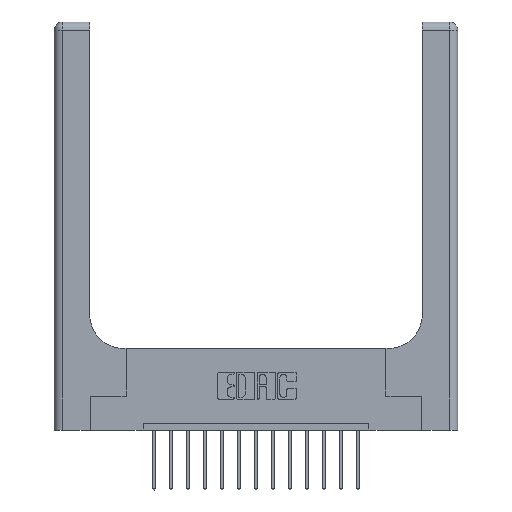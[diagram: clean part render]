
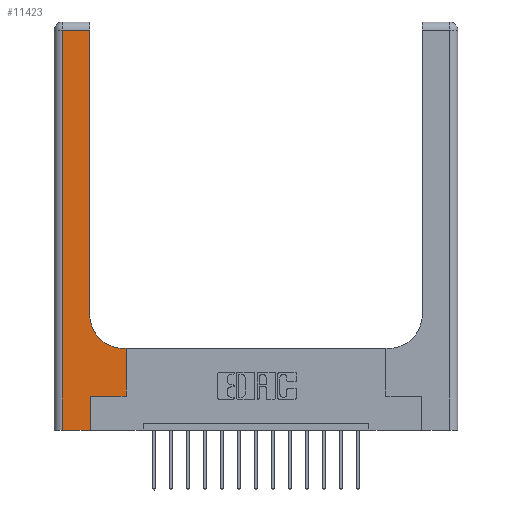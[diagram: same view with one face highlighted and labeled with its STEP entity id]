
A CAD part, top view. The second image highlights one B-rep face of the part: STEP entity #11423.
In plain terms, the highlighted planar face has unit normal (0, 0, 1).
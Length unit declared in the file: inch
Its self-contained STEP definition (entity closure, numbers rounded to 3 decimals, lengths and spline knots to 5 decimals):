
#412 = VERTEX_POINT ( 'NONE', #4691 ) ;
#681 = DIRECTION ( 'NONE',  ( 1., 0., 0. ) ) ;
#882 = LINE ( 'NONE', #3858, #10049 ) ;
#1026 = CARTESIAN_POINT ( 'NONE',  ( 0.528, 0.25, 0.37 ) ) ;
#1270 = DIRECTION ( 'NONE',  ( -1., 0., 0. ) ) ;
#1473 = ORIENTED_EDGE ( 'NONE', *, *, #4287, .T. ) ;
#1665 = DIRECTION ( 'NONE',  ( 0., 1., 0. ) ) ;
#1881 = CARTESIAN_POINT ( 'NONE',  ( 0.51, 0.85, 0.37 ) ) ;
#2483 = CARTESIAN_POINT ( 'NONE',  ( 0., 2.94, 0.37 ) ) ;
#3481 = PLANE ( 'NONE',  #8077 ) ;
#3617 = EDGE_LOOP ( 'NONE', ( #3775, #4340, #14629, #13721, #16088, #1473, #5250, #4185, #15981 ) ) ;
#3775 = ORIENTED_EDGE ( 'NONE', *, *, #16569, .T. ) ;
#3858 = CARTESIAN_POINT ( 'NONE',  ( 0., 0., 0.37 ) ) ;
#4105 = EDGE_CURVE ( 'NONE', #11452, #9670, #882, .T. ) ;
#4185 = ORIENTED_EDGE ( 'NONE', *, *, #8243, .T. ) ;
#4287 = EDGE_CURVE ( 'NONE', #4776, #412, #4812, .T. ) ;
#4327 = VECTOR ( 'NONE', #13483, 39.37008 ) ;
#4340 = ORIENTED_EDGE ( 'NONE', *, *, #14759, .T. ) ;
#4378 = DIRECTION ( 'NONE',  ( 1., 0., 0. ) ) ;
#4650 = FACE_OUTER_BOUND ( 'NONE', #3617, .T. ) ;
#4691 = CARTESIAN_POINT ( 'NONE',  ( 0.528, 0.25, 0.37 ) ) ;
#4776 = VERTEX_POINT ( 'NONE', #5897 ) ;
#4778 = CIRCLE ( 'NONE', #5193, 0.25 ) ;
#4812 = LINE ( 'NONE', #8342, #9183 ) ;
#5111 = DIRECTION ( 'NONE',  ( 0., 1., 0. ) ) ;
#5133 = LINE ( 'NONE', #13171, #6807 ) ;
#5193 = AXIS2_PLACEMENT_3D ( 'NONE', #1881, #7265, #681 ) ;
#5250 = ORIENTED_EDGE ( 'NONE', *, *, #8212, .T. ) ;
#5443 = DIRECTION ( 'NONE',  ( 0., 0., -1. ) ) ;
#5809 = LINE ( 'NONE', #8384, #4327 ) ;
#5897 = CARTESIAN_POINT ( 'NONE',  ( 0.265, 0.25, 0.37 ) ) ;
#6127 = EDGE_CURVE ( 'NONE', #13073, #7409, #4778, .T. ) ;
#6282 = DIRECTION ( 'NONE',  ( 1., 0., 0. ) ) ;
#6623 = DIRECTION ( 'NONE',  ( -1., 0., 0. ) ) ;
#6807 = VECTOR ( 'NONE', #14375, 39.37008 ) ;
#7076 = EDGE_CURVE ( 'NONE', #15290, #11452, #5809, .T. ) ;
#7146 = CARTESIAN_POINT ( 'NONE',  ( 0.26, 3., 0.37 ) ) ;
#7218 = VECTOR ( 'NONE', #5111, 39.37008 ) ;
#7265 = DIRECTION ( 'NONE',  ( 0., 0., -1. ) ) ;
#7409 = VERTEX_POINT ( 'NONE', #11857 ) ;
#7507 = CARTESIAN_POINT ( 'NONE',  ( 0.528, 0.6, 0.37 ) ) ;
#7717 = DIRECTION ( 'NONE',  ( 0., 1., 0. ) ) ;
#7907 = CARTESIAN_POINT ( 'NONE',  ( 0.265, 0., 0.37 ) ) ;
#8077 = AXIS2_PLACEMENT_3D ( 'NONE', #12709, #5443, #6623 ) ;
#8120 = VECTOR ( 'NONE', #1270, 39.37008 ) ;
#8212 = EDGE_CURVE ( 'NONE', #412, #8752, #16537, .T. ) ;
#8243 = EDGE_CURVE ( 'NONE', #8752, #13073, #5133, .T. ) ;
#8342 = CARTESIAN_POINT ( 'NONE',  ( 0.265, 0.25, 0.37 ) ) ;
#8384 = CARTESIAN_POINT ( 'NONE',  ( 0.06, 3., 0.37 ) ) ;
#8632 = VECTOR ( 'NONE', #7717, 39.37008 ) ;
#8752 = VERTEX_POINT ( 'NONE', #7507 ) ;
#9023 = EDGE_CURVE ( 'NONE', #9670, #4776, #12110, .T. ) ;
#9183 = VECTOR ( 'NONE', #4378, 39.37008 ) ;
#9670 = VERTEX_POINT ( 'NONE', #7907 ) ;
#10049 = VECTOR ( 'NONE', #6282, 39.37008 ) ;
#10621 = LINE ( 'NONE', #2483, #8120 ) ;
#11423 = ADVANCED_FACE ( 'NONE', ( #4650 ), #3481, .F. ) ;
#11452 = VERTEX_POINT ( 'NONE', #16045 ) ;
#11696 = CARTESIAN_POINT ( 'NONE',  ( 0.265, 0., 0.37 ) ) ;
#11857 = CARTESIAN_POINT ( 'NONE',  ( 0.26, 0.85, 0.37 ) ) ;
#12110 = LINE ( 'NONE', #11696, #8632 ) ;
#12173 = CARTESIAN_POINT ( 'NONE',  ( 0.51, 0.6, 0.37 ) ) ;
#12620 = CARTESIAN_POINT ( 'NONE',  ( 0.26, 2.94, 0.37 ) ) ;
#12709 = CARTESIAN_POINT ( 'NONE',  ( 0., 3., 0.37 ) ) ;
#13073 = VERTEX_POINT ( 'NONE', #12173 ) ;
#13171 = CARTESIAN_POINT ( 'NONE',  ( 0.26, 0.6, 0.37 ) ) ;
#13319 = LINE ( 'NONE', #7146, #14597 ) ;
#13483 = DIRECTION ( 'NONE',  ( 0., -1., 0. ) ) ;
#13721 = ORIENTED_EDGE ( 'NONE', *, *, #4105, .T. ) ;
#14375 = DIRECTION ( 'NONE',  ( -1., 0., 0. ) ) ;
#14597 = VECTOR ( 'NONE', #1665, 39.37008 ) ;
#14629 = ORIENTED_EDGE ( 'NONE', *, *, #7076, .T. ) ;
#14759 = EDGE_CURVE ( 'NONE', #15579, #15290, #10621, .T. ) ;
#15085 = CARTESIAN_POINT ( 'NONE',  ( 0.06, 2.94, 0.37 ) ) ;
#15290 = VERTEX_POINT ( 'NONE', #15085 ) ;
#15579 = VERTEX_POINT ( 'NONE', #12620 ) ;
#15981 = ORIENTED_EDGE ( 'NONE', *, *, #6127, .T. ) ;
#16045 = CARTESIAN_POINT ( 'NONE',  ( 0.06, 0., 0.37 ) ) ;
#16088 = ORIENTED_EDGE ( 'NONE', *, *, #9023, .T. ) ;
#16537 = LINE ( 'NONE', #1026, #7218 ) ;
#16569 = EDGE_CURVE ( 'NONE', #7409, #15579, #13319, .T. ) ;
